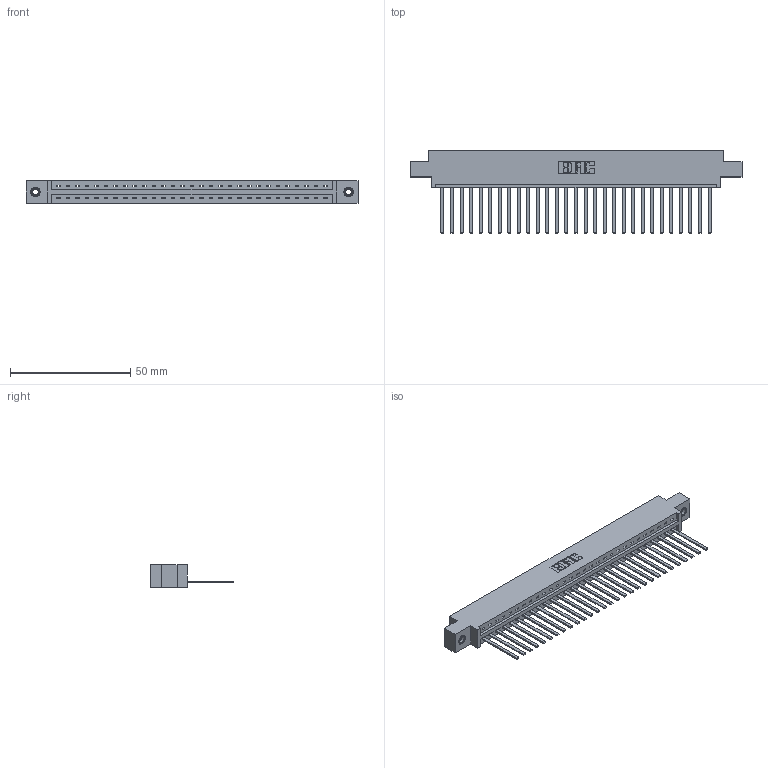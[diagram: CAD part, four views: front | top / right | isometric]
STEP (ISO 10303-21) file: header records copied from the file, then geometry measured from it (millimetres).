
FILE_DESCRIPTION (( 'STEP AP203' ), '1' );
FILE_NAME ('337-029-544-607.STEP', '2019-09-30T22:51:19', ( '' ), ( '' ), 'SwSTEP 2.0', 'SolidWorks 2016', '' );
FILE_SCHEMA (( 'CONFIG_CONTROL_DESIGN' ));
Length unit declared in the file: inch
Products named in the file (4): 337-029-544-607; 345-250-001_345-250-005-103; 345-292-001_345-293-144; 337 Part_0.170 Offset - 0.156 Dia-TI
Assembly tree (32 placements, depth 2):
  337-029-544-607
    337 Part_0.170 Offset - 0.156 Dia-TI
    345-292-001_345-293-144  x29
    345-250-001_345-250-005-103  x2
Bounding box: 137.92 x 34.3 x 9.4 mm (x, y, z)
Volume: 14376.8 mm3; surface area: 16026.5 mm2
Topology: 32 solids, 32 shells, 1802 faces, 5389 edges, 3546 vertices
Faces by surface type: plane 1324, cylinder 462, cone 12, torus 4
Entity records: 24372 total; most frequent: CARTESIAN_POINT 4224, ORIENTED_EDGE 4182, DIRECTION 3611, EDGE_CURVE 2091, LINE 1947, VECTOR 1947, VERTEX_POINT 1388, AXIS2_PLACEMENT_3D 832
